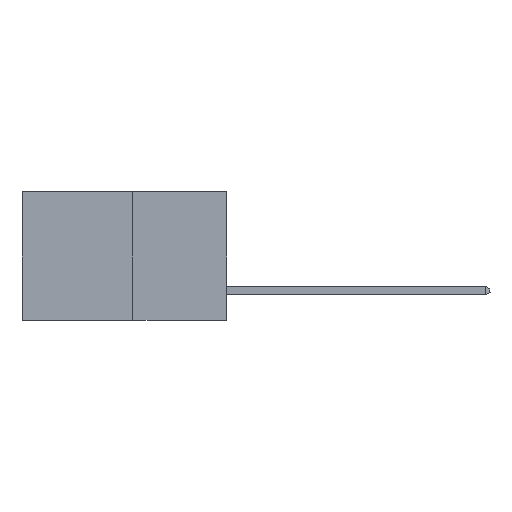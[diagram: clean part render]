
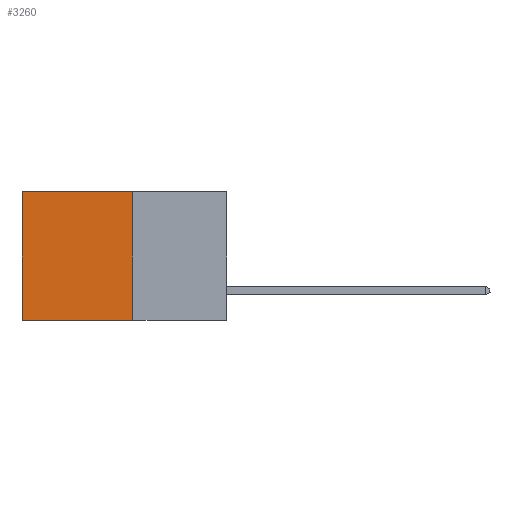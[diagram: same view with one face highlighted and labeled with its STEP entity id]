
A CAD part, left-side view. The second image highlights one B-rep face of the part: STEP entity #3260.
In plain terms, the highlighted planar face has unit normal (-1, 0, 0).
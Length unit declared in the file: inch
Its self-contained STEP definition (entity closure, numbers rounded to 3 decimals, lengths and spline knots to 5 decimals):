
#500 = EDGE_CURVE ( 'NONE', #7977, #27380, #28286, .T. ) ;
#737 = CARTESIAN_POINT ( 'NONE',  ( 0.277, 0.27, 0. ) ) ;
#934 = CARTESIAN_POINT ( 'NONE',  ( 0.277, 0.27, 0. ) ) ;
#1025 = CARTESIAN_POINT ( 'NONE',  ( 0.277, 0.59, 0. ) ) ;
#3260 = ADVANCED_FACE ( 'NONE', ( #17300 ), #10254, .F. ) ;
#3292 = DIRECTION ( 'NONE',  ( 0., 1., 0. ) ) ;
#4391 = VECTOR ( 'NONE', #13139, 39.37008 ) ;
#5571 = LINE ( 'NONE', #934, #17207 ) ;
#6010 = DIRECTION ( 'NONE',  ( 0., 1., 0. ) ) ;
#6030 = CARTESIAN_POINT ( 'NONE',  ( 0.277, 0.59, -0.37 ) ) ;
#7015 = VERTEX_POINT ( 'NONE', #737 ) ;
#7977 = VERTEX_POINT ( 'NONE', #1025 ) ;
#10254 = PLANE ( 'NONE',  #16994 ) ;
#10726 = DIRECTION ( 'NONE',  ( 0., 0., -1. ) ) ;
#10768 = CARTESIAN_POINT ( 'NONE',  ( 0.277, 0.27, -0.37 ) ) ;
#10781 = ORIENTED_EDGE ( 'NONE', *, *, #500, .T. ) ;
#11805 = VECTOR ( 'NONE', #6010, 39.37008 ) ;
#13092 = CARTESIAN_POINT ( 'NONE',  ( 0.277, 0.59, -0.37 ) ) ;
#13139 = DIRECTION ( 'NONE',  ( 0., 0., -1. ) ) ;
#13303 = LINE ( 'NONE', #26812, #11805 ) ;
#14942 = DIRECTION ( 'NONE',  ( 0., 0., -1. ) ) ;
#16810 = ORIENTED_EDGE ( 'NONE', *, *, #29633, .F. ) ;
#16994 = AXIS2_PLACEMENT_3D ( 'NONE', #26496, #28819, #14942 ) ;
#17207 = VECTOR ( 'NONE', #3292, 39.37008 ) ;
#17300 = FACE_OUTER_BOUND ( 'NONE', #18995, .T. ) ;
#18995 = EDGE_LOOP ( 'NONE', ( #10781, #16810, #25176, #22260 ) ) ;
#20543 = EDGE_CURVE ( 'NONE', #7015, #7977, #5571, .T. ) ;
#22085 = EDGE_CURVE ( 'NONE', #7015, #27882, #22911, .T. ) ;
#22260 = ORIENTED_EDGE ( 'NONE', *, *, #20543, .T. ) ;
#22911 = LINE ( 'NONE', #10768, #4391 ) ;
#25176 = ORIENTED_EDGE ( 'NONE', *, *, #22085, .F. ) ;
#26496 = CARTESIAN_POINT ( 'NONE',  ( 0.277, 0.27, -0.37 ) ) ;
#26513 = CARTESIAN_POINT ( 'NONE',  ( 0.277, 0.27, -0.37 ) ) ;
#26812 = CARTESIAN_POINT ( 'NONE',  ( 0.277, 0.27, -0.37 ) ) ;
#27380 = VERTEX_POINT ( 'NONE', #13092 ) ;
#27882 = VERTEX_POINT ( 'NONE', #26513 ) ;
#28286 = LINE ( 'NONE', #6030, #29030 ) ;
#28819 = DIRECTION ( 'NONE',  ( 1., 0., 0. ) ) ;
#29030 = VECTOR ( 'NONE', #10726, 39.37008 ) ;
#29633 = EDGE_CURVE ( 'NONE', #27882, #27380, #13303, .T. ) ;
